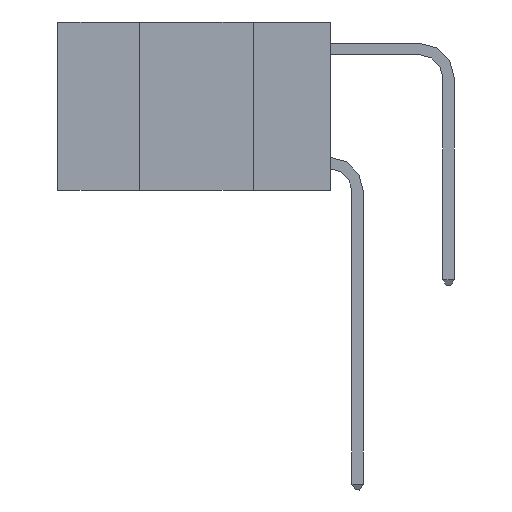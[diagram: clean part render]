
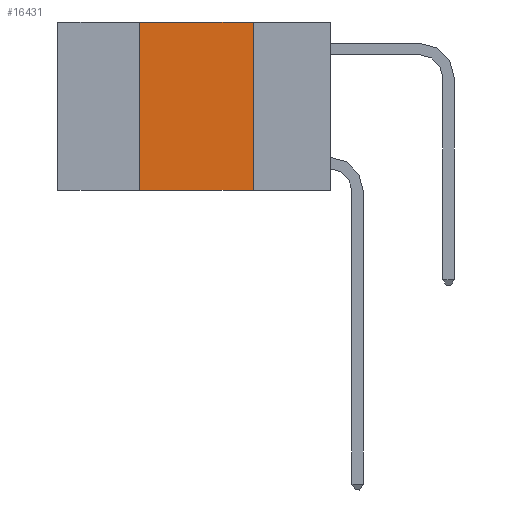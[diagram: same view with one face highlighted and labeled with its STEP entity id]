
A CAD part, left-side view. The second image highlights one B-rep face of the part: STEP entity #16431.
In plain terms, the highlighted planar face has unit normal (-1, 0, 0).
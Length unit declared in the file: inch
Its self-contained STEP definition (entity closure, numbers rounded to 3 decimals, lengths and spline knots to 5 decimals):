
#2092 = EDGE_CURVE ( 'NONE', #18501, #21258, #11962, .T. ) ;
#2776 = DIRECTION ( 'NONE',  ( 0., -1., 0. ) ) ;
#2882 = DIRECTION ( 'NONE',  ( 0., 0., 1. ) ) ;
#2929 = PLANE ( 'NONE',  #16720 ) ;
#5295 = FACE_OUTER_BOUND ( 'NONE', #21924, .T. ) ;
#5442 = CARTESIAN_POINT ( 'NONE',  ( 0., 0.6, 0. ) ) ;
#5747 = LINE ( 'NONE', #10105, #32944 ) ;
#7907 = LINE ( 'NONE', #33208, #21138 ) ;
#8116 = ORIENTED_EDGE ( 'NONE', *, *, #32752, .T. ) ;
#10105 = CARTESIAN_POINT ( 'NONE',  ( 0., 0.17, 0. ) ) ;
#10353 = VECTOR ( 'NONE', #2882, 39.37008 ) ;
#10874 = DIRECTION ( 'NONE',  ( 1., 0., 0. ) ) ;
#11790 = CARTESIAN_POINT ( 'NONE',  ( 0., 0.17, 0. ) ) ;
#11962 = LINE ( 'NONE', #5442, #32185 ) ;
#13476 = ORIENTED_EDGE ( 'NONE', *, *, #33080, .F. ) ;
#15247 = CARTESIAN_POINT ( 'NONE',  ( 0., 0.17, -0.37 ) ) ;
#15406 = DIRECTION ( 'NONE',  ( 0., 0., -1. ) ) ;
#16198 = EDGE_CURVE ( 'NONE', #21258, #34075, #5747, .T. ) ;
#16431 = ADVANCED_FACE ( 'NONE', ( #5295 ), #2929, .F. ) ;
#16720 = AXIS2_PLACEMENT_3D ( 'NONE', #26664, #10874, #29314 ) ;
#18294 = VERTEX_POINT ( 'NONE', #28866 ) ;
#18501 = VERTEX_POINT ( 'NONE', #24488 ) ;
#20080 = DIRECTION ( 'NONE',  ( 0., -1., 0. ) ) ;
#21138 = VECTOR ( 'NONE', #20080, 39.37008 ) ;
#21258 = VERTEX_POINT ( 'NONE', #11790 ) ;
#21924 = EDGE_LOOP ( 'NONE', ( #32038, #26673, #13476, #8116 ) ) ;
#24488 = CARTESIAN_POINT ( 'NONE',  ( 0., 0.42, 0. ) ) ;
#25220 = LINE ( 'NONE', #26497, #10353 ) ;
#26497 = CARTESIAN_POINT ( 'NONE',  ( 0., 0.42, 0. ) ) ;
#26664 = CARTESIAN_POINT ( 'NONE',  ( 0., 0.6, 0. ) ) ;
#26673 = ORIENTED_EDGE ( 'NONE', *, *, #2092, .F. ) ;
#28866 = CARTESIAN_POINT ( 'NONE',  ( 0., 0.42, -0.37 ) ) ;
#29314 = DIRECTION ( 'NONE',  ( 0., 0., -1. ) ) ;
#32038 = ORIENTED_EDGE ( 'NONE', *, *, #16198, .F. ) ;
#32185 = VECTOR ( 'NONE', #2776, 39.37008 ) ;
#32752 = EDGE_CURVE ( 'NONE', #18294, #34075, #7907, .T. ) ;
#32944 = VECTOR ( 'NONE', #15406, 39.37008 ) ;
#33080 = EDGE_CURVE ( 'NONE', #18294, #18501, #25220, .T. ) ;
#33208 = CARTESIAN_POINT ( 'NONE',  ( 0., 0.6, -0.37 ) ) ;
#34075 = VERTEX_POINT ( 'NONE', #15247 ) ;
